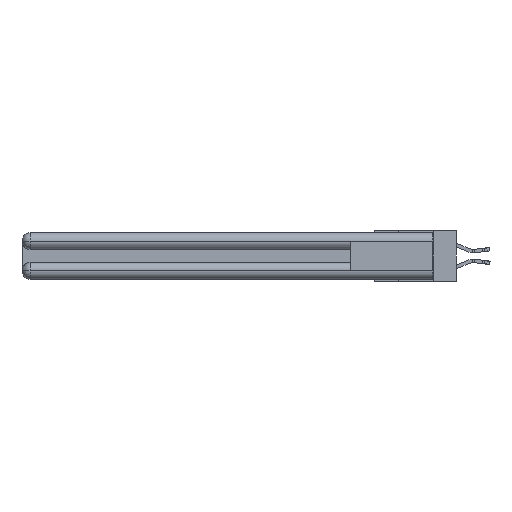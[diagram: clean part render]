
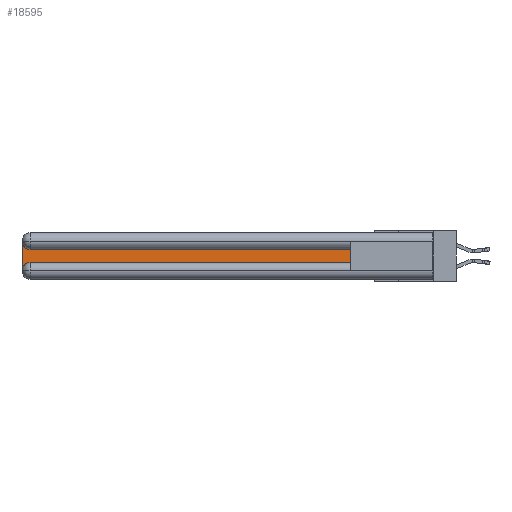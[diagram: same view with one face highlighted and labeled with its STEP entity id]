
A CAD part, left-side view. The second image highlights one B-rep face of the part: STEP entity #18595.
In plain terms, the highlighted planar face has unit normal (-1, 0, 0).
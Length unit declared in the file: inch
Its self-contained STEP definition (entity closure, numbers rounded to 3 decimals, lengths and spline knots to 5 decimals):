
#268 = CARTESIAN_POINT ( 'NONE',  ( 0.075, 2.94, -0.2175 ) ) ;
#349 = ORIENTED_EDGE ( 'NONE', *, *, #23724, .T. ) ;
#621 = ORIENTED_EDGE ( 'NONE', *, *, #2743, .T. ) ;
#924 = FACE_OUTER_BOUND ( 'NONE', #6505, .T. ) ;
#1262 = CARTESIAN_POINT ( 'NONE',  ( 0.075, 3., -0.1225 ) ) ;
#2743 = EDGE_CURVE ( 'NONE', #3859, #27728, #18995, .T. ) ;
#3473 = AXIS2_PLACEMENT_3D ( 'NONE', #1262, #16980, #14865 ) ;
#3656 = DIRECTION ( 'NONE',  ( 0., -1., 0. ) ) ;
#3859 = VERTEX_POINT ( 'NONE', #28765 ) ;
#4235 = LINE ( 'NONE', #26416, #14692 ) ;
#4912 = ORIENTED_EDGE ( 'NONE', *, *, #23767, .T. ) ;
#5652 = ORIENTED_EDGE ( 'NONE', *, *, #23687, .T. ) ;
#5677 = VERTEX_POINT ( 'NONE', #27182 ) ;
#6206 = VECTOR ( 'NONE', #24365, 39.37008 ) ;
#6505 = EDGE_LOOP ( 'NONE', ( #24314, #621, #5652, #4912, #349, #22785 ) ) ;
#8384 = VECTOR ( 'NONE', #28162, 39.37008 ) ;
#8801 = DIRECTION ( 'NONE',  ( 1., 0., 0. ) ) ;
#10141 = VECTOR ( 'NONE', #3656, 39.37008 ) ;
#11073 = AXIS2_PLACEMENT_3D ( 'NONE', #24083, #14978, #14685 ) ;
#11135 = VERTEX_POINT ( 'NONE', #17106 ) ;
#12007 = VERTEX_POINT ( 'NONE', #25071 ) ;
#12215 = CARTESIAN_POINT ( 'NONE',  ( 0.075, 0.6, -0.2175 ) ) ;
#12321 = LINE ( 'NONE', #26872, #6206 ) ;
#13585 = AXIS2_PLACEMENT_3D ( 'NONE', #17972, #8801, #27068 ) ;
#13796 = LINE ( 'NONE', #12215, #8384 ) ;
#13992 = VERTEX_POINT ( 'NONE', #268 ) ;
#14685 = DIRECTION ( 'NONE',  ( 0., 0., -1. ) ) ;
#14692 = VECTOR ( 'NONE', #14884, 39.37008 ) ;
#14865 = DIRECTION ( 'NONE',  ( 0., 0., -1. ) ) ;
#14884 = DIRECTION ( 'NONE',  ( 0., 1., 0. ) ) ;
#14978 = DIRECTION ( 'NONE',  ( 1., 0., 0. ) ) ;
#15211 = CIRCLE ( 'NONE', #13585, 0.06 ) ;
#16980 = DIRECTION ( 'NONE',  ( 1., 0., 0. ) ) ;
#17106 = CARTESIAN_POINT ( 'NONE',  ( 0.075, 0.6, -0.1225 ) ) ;
#17455 = CARTESIAN_POINT ( 'NONE',  ( 0.075, 0.6, -0.2175 ) ) ;
#17972 = CARTESIAN_POINT ( 'NONE',  ( 0.075, 2.94, -0.2775 ) ) ;
#18595 = ADVANCED_FACE ( 'NONE', ( #924 ), #19444, .F. ) ;
#18995 = CIRCLE ( 'NONE', #11073, 0.06 ) ;
#19444 = PLANE ( 'NONE',  #3473 ) ;
#20755 = EDGE_CURVE ( 'NONE', #11135, #3859, #4235, .T. ) ;
#21430 = LINE ( 'NONE', #17455, #10141 ) ;
#22785 = ORIENTED_EDGE ( 'NONE', *, *, #28364, .T. ) ;
#23687 = EDGE_CURVE ( 'NONE', #27728, #5677, #12321, .T. ) ;
#23724 = EDGE_CURVE ( 'NONE', #13992, #12007, #21430, .T. ) ;
#23767 = EDGE_CURVE ( 'NONE', #5677, #13992, #15211, .T. ) ;
#24083 = CARTESIAN_POINT ( 'NONE',  ( 0.075, 2.94, -0.0625 ) ) ;
#24314 = ORIENTED_EDGE ( 'NONE', *, *, #20755, .T. ) ;
#24365 = DIRECTION ( 'NONE',  ( 0., 0., -1. ) ) ;
#24514 = CARTESIAN_POINT ( 'NONE',  ( 0.075, 3., -0.0625 ) ) ;
#25071 = CARTESIAN_POINT ( 'NONE',  ( 0.075, 0.6, -0.2175 ) ) ;
#26416 = CARTESIAN_POINT ( 'NONE',  ( 0.075, 0.6, -0.1225 ) ) ;
#26872 = CARTESIAN_POINT ( 'NONE',  ( 0.075, 3., -0.2175 ) ) ;
#27068 = DIRECTION ( 'NONE',  ( 0., 0., -1. ) ) ;
#27182 = CARTESIAN_POINT ( 'NONE',  ( 0.075, 3., -0.2775 ) ) ;
#27728 = VERTEX_POINT ( 'NONE', #24514 ) ;
#28162 = DIRECTION ( 'NONE',  ( 0., 0., 1. ) ) ;
#28364 = EDGE_CURVE ( 'NONE', #12007, #11135, #13796, .T. ) ;
#28765 = CARTESIAN_POINT ( 'NONE',  ( 0.075, 2.94, -0.1225 ) ) ;
